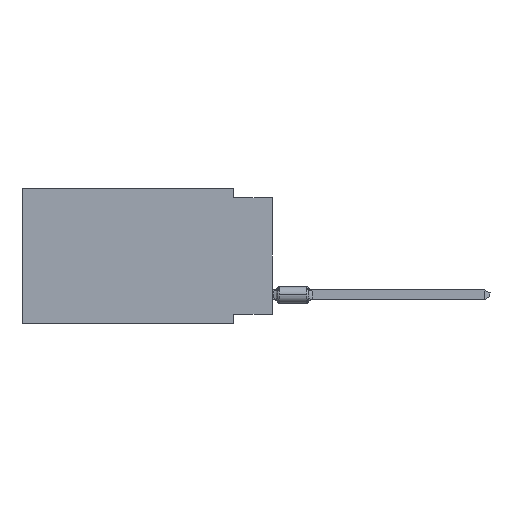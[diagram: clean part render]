
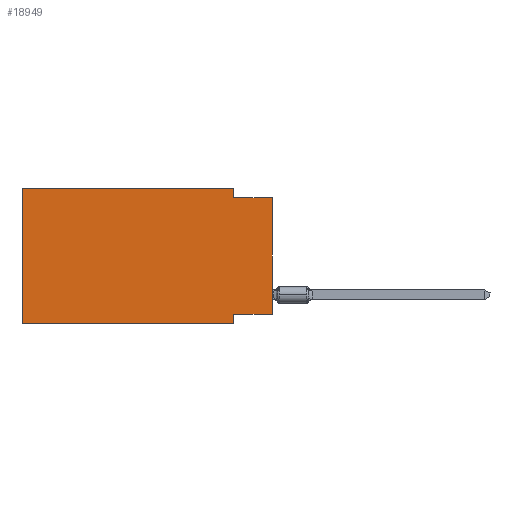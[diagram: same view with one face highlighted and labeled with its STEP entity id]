
A CAD part, left-side view. The second image highlights one B-rep face of the part: STEP entity #18949.
In plain terms, the highlighted planar face has unit normal (-1, 0, 0).
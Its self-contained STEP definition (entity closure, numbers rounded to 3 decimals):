
#344 = CARTESIAN_POINT ( 'NONE',  ( 0., 16.383, -8.89 ) ) ;
#397 = CARTESIAN_POINT ( 'NONE',  ( 0., 16.383, 0. ) ) ;
#1490 = ORIENTED_EDGE ( 'NONE', *, *, #20324, .F. ) ;
#1801 = EDGE_CURVE ( 'NONE', #39790, #11011, #23643, .T. ) ;
#1971 = EDGE_CURVE ( 'NONE', #3323, #28155, #5364, .T. ) ;
#2228 = DIRECTION ( 'NONE',  ( 0., 0., 1. ) ) ;
#2313 = VECTOR ( 'NONE', #28254, 1000. ) ;
#3315 = CARTESIAN_POINT ( 'NONE',  ( 0., 2.54, -8.89 ) ) ;
#3323 = VERTEX_POINT ( 'NONE', #344 ) ;
#3439 = VECTOR ( 'NONE', #9856, 1000. ) ;
#5280 = CARTESIAN_POINT ( 'NONE',  ( 0., 2.54, -0.635 ) ) ;
#5328 = ORIENTED_EDGE ( 'NONE', *, *, #30403, .F. ) ;
#5364 = LINE ( 'NONE', #48918, #3439 ) ;
#6068 = CARTESIAN_POINT ( 'NONE',  ( 0., 0., -0.635 ) ) ;
#8446 = LINE ( 'NONE', #51994, #47587 ) ;
#8508 = FACE_OUTER_BOUND ( 'NONE', #35206, .T. ) ;
#9290 = DIRECTION ( 'NONE',  ( 0., -1., 0. ) ) ;
#9856 = DIRECTION ( 'NONE',  ( 0., -1., 0. ) ) ;
#10721 = AXIS2_PLACEMENT_3D ( 'NONE', #24466, #47878, #38890 ) ;
#11011 = VERTEX_POINT ( 'NONE', #5280 ) ;
#11635 = ORIENTED_EDGE ( 'NONE', *, *, #28331, .F. ) ;
#11909 = CARTESIAN_POINT ( 'NONE',  ( 0., 2.54, -8.255 ) ) ;
#12825 = VERTEX_POINT ( 'NONE', #51047 ) ;
#13658 = ORIENTED_EDGE ( 'NONE', *, *, #53109, .F. ) ;
#14459 = LINE ( 'NONE', #397, #38477 ) ;
#15876 = VERTEX_POINT ( 'NONE', #59939 ) ;
#18714 = PLANE ( 'NONE',  #10721 ) ;
#18949 = ADVANCED_FACE ( 'NONE', ( #8508 ), #18714, .F. ) ;
#19191 = LINE ( 'NONE', #57335, #47814 ) ;
#19890 = DIRECTION ( 'NONE',  ( 0., 0., 1. ) ) ;
#20324 = EDGE_CURVE ( 'NONE', #3323, #12825, #14459, .T. ) ;
#22222 = DIRECTION ( 'NONE',  ( 0., -1., 0. ) ) ;
#23364 = VERTEX_POINT ( 'NONE', #11909 ) ;
#23643 = LINE ( 'NONE', #24265, #59683 ) ;
#23908 = VECTOR ( 'NONE', #2228, 1000. ) ;
#24265 = CARTESIAN_POINT ( 'NONE',  ( 0., 2.54, 0. ) ) ;
#24316 = LINE ( 'NONE', #43550, #40190 ) ;
#24466 = CARTESIAN_POINT ( 'NONE',  ( 0., 16.383, 0. ) ) ;
#28155 = VERTEX_POINT ( 'NONE', #38898 ) ;
#28254 = DIRECTION ( 'NONE',  ( 0., 0., -1. ) ) ;
#28331 = EDGE_CURVE ( 'NONE', #12825, #39790, #8446, .T. ) ;
#30403 = EDGE_CURVE ( 'NONE', #15876, #23364, #19191, .T. ) ;
#30725 = ORIENTED_EDGE ( 'NONE', *, *, #36859, .T. ) ;
#32637 = DIRECTION ( 'NONE',  ( 0., 0., -1. ) ) ;
#35206 = EDGE_LOOP ( 'NONE', ( #30725, #50059, #57090, #11635, #1490, #43353, #13658, #5328 ) ) ;
#36818 = CARTESIAN_POINT ( 'NONE',  ( 0., 0., 0. ) ) ;
#36859 = EDGE_CURVE ( 'NONE', #15876, #56590, #51203, .T. ) ;
#38477 = VECTOR ( 'NONE', #19890, 1000. ) ;
#38890 = DIRECTION ( 'NONE',  ( 0., 0., -1. ) ) ;
#38898 = CARTESIAN_POINT ( 'NONE',  ( 0., 2.54, -8.89 ) ) ;
#39790 = VERTEX_POINT ( 'NONE', #45742 ) ;
#40190 = VECTOR ( 'NONE', #9290, 1000. ) ;
#43353 = ORIENTED_EDGE ( 'NONE', *, *, #1971, .T. ) ;
#43550 = CARTESIAN_POINT ( 'NONE',  ( 0., 0., -0.635 ) ) ;
#45742 = CARTESIAN_POINT ( 'NONE',  ( 0., 2.54, 0. ) ) ;
#47587 = VECTOR ( 'NONE', #22222, 1000. ) ;
#47814 = VECTOR ( 'NONE', #60148, 1000. ) ;
#47878 = DIRECTION ( 'NONE',  ( 1., 0., 0. ) ) ;
#48918 = CARTESIAN_POINT ( 'NONE',  ( 0., 16.383, -8.89 ) ) ;
#50059 = ORIENTED_EDGE ( 'NONE', *, *, #57891, .F. ) ;
#51047 = CARTESIAN_POINT ( 'NONE',  ( 0., 16.383, 0. ) ) ;
#51203 = LINE ( 'NONE', #36818, #23908 ) ;
#51994 = CARTESIAN_POINT ( 'NONE',  ( 0., 16.383, 0. ) ) ;
#52278 = LINE ( 'NONE', #3315, #2313 ) ;
#53109 = EDGE_CURVE ( 'NONE', #23364, #28155, #52278, .T. ) ;
#56590 = VERTEX_POINT ( 'NONE', #6068 ) ;
#57090 = ORIENTED_EDGE ( 'NONE', *, *, #1801, .F. ) ;
#57335 = CARTESIAN_POINT ( 'NONE',  ( 0., 0., -8.255 ) ) ;
#57891 = EDGE_CURVE ( 'NONE', #11011, #56590, #24316, .T. ) ;
#59683 = VECTOR ( 'NONE', #32637, 1000. ) ;
#59939 = CARTESIAN_POINT ( 'NONE',  ( 0., 0., -8.255 ) ) ;
#60148 = DIRECTION ( 'NONE',  ( 0., 1., 0. ) ) ;
